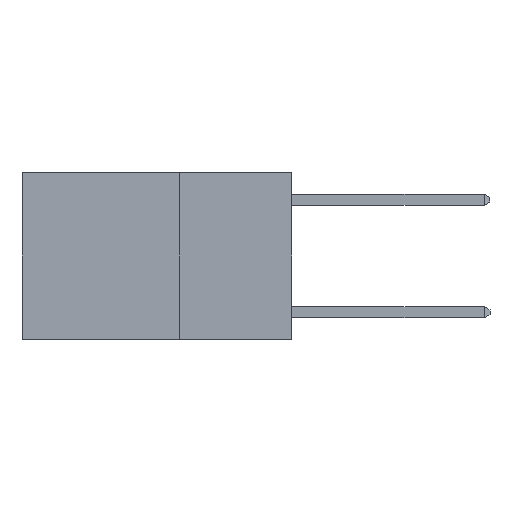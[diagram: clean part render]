
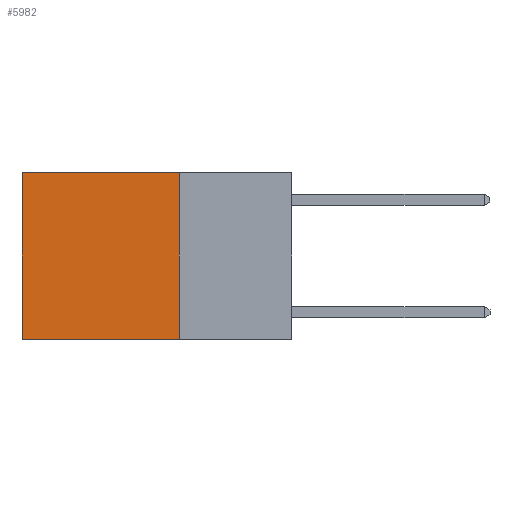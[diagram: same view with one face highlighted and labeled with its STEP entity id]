
A CAD part, left-side view. The second image highlights one B-rep face of the part: STEP entity #5982.
In plain terms, the highlighted planar face has unit normal (-1, 0, 0).
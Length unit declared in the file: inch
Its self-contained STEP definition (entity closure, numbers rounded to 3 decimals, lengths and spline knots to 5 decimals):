
#116 = CARTESIAN_POINT ( 'NONE',  ( 0.2625, 0.6, 0. ) ) ;
#305 = DIRECTION ( 'NONE',  ( 1., 0., 0. ) ) ;
#565 = DIRECTION ( 'NONE',  ( 0., 1., 0. ) ) ;
#712 = ORIENTED_EDGE ( 'NONE', *, *, #7512, .T. ) ;
#885 = LINE ( 'NONE', #116, #7023 ) ;
#1108 = CARTESIAN_POINT ( 'NONE',  ( 0.2625, 0.6, -0.37 ) ) ;
#1734 = DIRECTION ( 'NONE',  ( 0., 0., -1. ) ) ;
#1808 = FACE_OUTER_BOUND ( 'NONE', #4975, .T. ) ;
#1881 = VERTEX_POINT ( 'NONE', #8130 ) ;
#3097 = CARTESIAN_POINT ( 'NONE',  ( 0.2625, 0.25, 0. ) ) ;
#3206 = VECTOR ( 'NONE', #3919, 39.37008 ) ;
#3526 = CARTESIAN_POINT ( 'NONE',  ( 0.2625, 0.25, 0. ) ) ;
#3692 = LINE ( 'NONE', #4582, #7689 ) ;
#3919 = DIRECTION ( 'NONE',  ( 0., 1., 0. ) ) ;
#4335 = VECTOR ( 'NONE', #8252, 39.37008 ) ;
#4582 = CARTESIAN_POINT ( 'NONE',  ( 0.2625, 0.25, -0.37 ) ) ;
#4961 = CARTESIAN_POINT ( 'NONE',  ( 0.2625, 0.6, 0. ) ) ;
#4975 = EDGE_LOOP ( 'NONE', ( #7799, #9520, #9893, #712 ) ) ;
#5104 = PLANE ( 'NONE',  #8018 ) ;
#5881 = DIRECTION ( 'NONE',  ( 0., 0., -1. ) ) ;
#5982 = ADVANCED_FACE ( 'NONE', ( #1808 ), #5104, .F. ) ;
#6450 = VERTEX_POINT ( 'NONE', #4961 ) ;
#7023 = VECTOR ( 'NONE', #1734, 39.37008 ) ;
#7128 = EDGE_CURVE ( 'NONE', #1881, #10142, #7207, .T. ) ;
#7207 = LINE ( 'NONE', #8294, #4335 ) ;
#7457 = LINE ( 'NONE', #3097, #3206 ) ;
#7512 = EDGE_CURVE ( 'NONE', #1881, #6450, #7457, .T. ) ;
#7689 = VECTOR ( 'NONE', #565, 39.37008 ) ;
#7799 = ORIENTED_EDGE ( 'NONE', *, *, #10231, .T. ) ;
#8018 = AXIS2_PLACEMENT_3D ( 'NONE', #3526, #305, #5881 ) ;
#8130 = CARTESIAN_POINT ( 'NONE',  ( 0.2625, 0.25, 0. ) ) ;
#8252 = DIRECTION ( 'NONE',  ( 0., 0., -1. ) ) ;
#8294 = CARTESIAN_POINT ( 'NONE',  ( 0.2625, 0.25, 0. ) ) ;
#8531 = VERTEX_POINT ( 'NONE', #1108 ) ;
#8885 = CARTESIAN_POINT ( 'NONE',  ( 0.2625, 0.25, -0.37 ) ) ;
#9520 = ORIENTED_EDGE ( 'NONE', *, *, #9940, .F. ) ;
#9893 = ORIENTED_EDGE ( 'NONE', *, *, #7128, .F. ) ;
#9940 = EDGE_CURVE ( 'NONE', #10142, #8531, #3692, .T. ) ;
#10142 = VERTEX_POINT ( 'NONE', #8885 ) ;
#10231 = EDGE_CURVE ( 'NONE', #6450, #8531, #885, .T. ) ;
